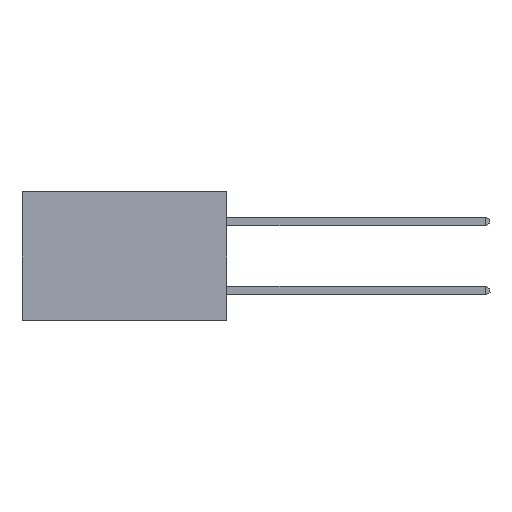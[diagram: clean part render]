
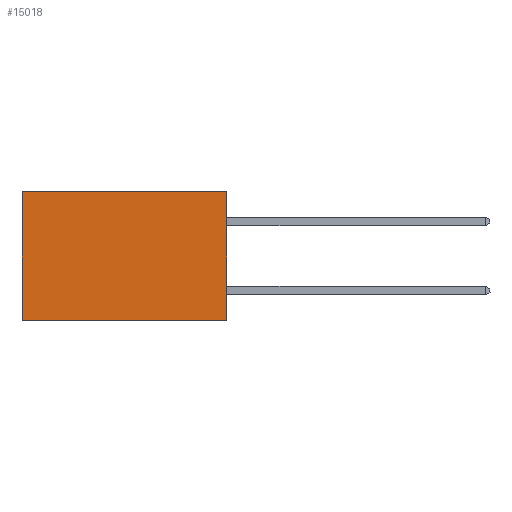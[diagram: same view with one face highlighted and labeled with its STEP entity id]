
A CAD part, left-side view. The second image highlights one B-rep face of the part: STEP entity #15018.
In plain terms, the highlighted planar face has unit normal (-1, 0, 0).
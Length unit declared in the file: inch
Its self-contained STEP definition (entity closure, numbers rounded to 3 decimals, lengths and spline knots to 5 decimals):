
#1092 = DIRECTION ( 'NONE',  ( 1., 0., 0. ) ) ;
#1430 = LINE ( 'NONE', #20113, #19529 ) ;
#2512 = ORIENTED_EDGE ( 'NONE', *, *, #16626, .F. ) ;
#3531 = CARTESIAN_POINT ( 'NONE',  ( 0.277, 0., 0. ) ) ;
#4610 = LINE ( 'NONE', #22352, #23385 ) ;
#5862 = CARTESIAN_POINT ( 'NONE',  ( 0.277, 0.59, -0.37 ) ) ;
#6080 = ORIENTED_EDGE ( 'NONE', *, *, #24215, .F. ) ;
#6755 = FACE_OUTER_BOUND ( 'NONE', #30902, .T. ) ;
#8522 = PLANE ( 'NONE',  #10558 ) ;
#8665 = EDGE_CURVE ( 'NONE', #30920, #24344, #20907, .T. ) ;
#10167 = CARTESIAN_POINT ( 'NONE',  ( 0.277, 0.59, -0.37 ) ) ;
#10558 = AXIS2_PLACEMENT_3D ( 'NONE', #15862, #1092, #18326 ) ;
#11717 = VERTEX_POINT ( 'NONE', #17425 ) ;
#11729 = EDGE_CURVE ( 'NONE', #18081, #30920, #4610, .T. ) ;
#12668 = DIRECTION ( 'NONE',  ( 0., 1., 0. ) ) ;
#14495 = CARTESIAN_POINT ( 'NONE',  ( 0.277, 0., -0.37 ) ) ;
#15018 = ADVANCED_FACE ( 'NONE', ( #6755 ), #8522, .F. ) ;
#15862 = CARTESIAN_POINT ( 'NONE',  ( 0.277, 0., -0.37 ) ) ;
#16626 = EDGE_CURVE ( 'NONE', #18081, #11717, #24227, .T. ) ;
#17425 = CARTESIAN_POINT ( 'NONE',  ( 0.277, 0., -0.37 ) ) ;
#17658 = CARTESIAN_POINT ( 'NONE',  ( 0.277, 0.59, 0. ) ) ;
#18081 = VERTEX_POINT ( 'NONE', #3531 ) ;
#18326 = DIRECTION ( 'NONE',  ( 0., 0., -1. ) ) ;
#19356 = VECTOR ( 'NONE', #22313, 39.37008 ) ;
#19529 = VECTOR ( 'NONE', #29685, 39.37008 ) ;
#20113 = CARTESIAN_POINT ( 'NONE',  ( 0.277, 0., -0.37 ) ) ;
#20781 = ORIENTED_EDGE ( 'NONE', *, *, #8665, .T. ) ;
#20907 = LINE ( 'NONE', #10167, #19356 ) ;
#21855 = DIRECTION ( 'NONE',  ( 0., 0., -1. ) ) ;
#22313 = DIRECTION ( 'NONE',  ( 0., 0., -1. ) ) ;
#22352 = CARTESIAN_POINT ( 'NONE',  ( 0.277, 0., 0. ) ) ;
#23385 = VECTOR ( 'NONE', #12668, 39.37008 ) ;
#24215 = EDGE_CURVE ( 'NONE', #11717, #24344, #1430, .T. ) ;
#24227 = LINE ( 'NONE', #14495, #29819 ) ;
#24344 = VERTEX_POINT ( 'NONE', #5862 ) ;
#29685 = DIRECTION ( 'NONE',  ( 0., 1., 0. ) ) ;
#29819 = VECTOR ( 'NONE', #21855, 39.37008 ) ;
#29858 = ORIENTED_EDGE ( 'NONE', *, *, #11729, .T. ) ;
#30902 = EDGE_LOOP ( 'NONE', ( #20781, #6080, #2512, #29858 ) ) ;
#30920 = VERTEX_POINT ( 'NONE', #17658 ) ;
